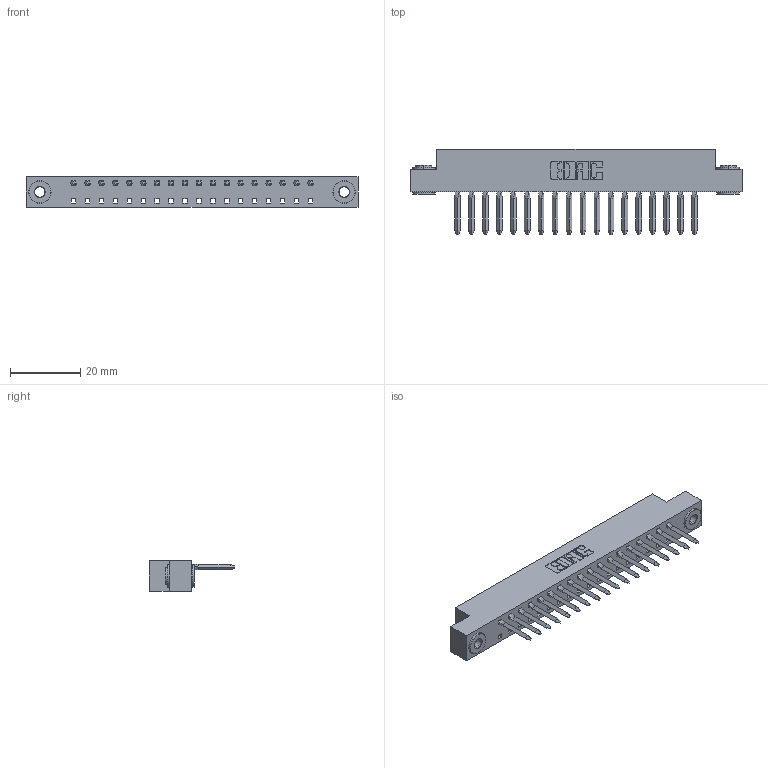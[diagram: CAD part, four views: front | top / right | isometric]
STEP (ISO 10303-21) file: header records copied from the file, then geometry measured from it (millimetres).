
FILE_DESCRIPTION (( 'STEP AP203' ), '1' );
FILE_NAME ('338-018-540-103.STEP', '2020-03-24T17:13:19', ( '' ), ( '' ), 'SwSTEP 2.0', 'SolidWorks 2016', '' );
FILE_SCHEMA (( 'CONFIG_CONTROL_DESIGN' ));
Length unit declared in the file: inch
Products named in the file (4): 338-290-001_540; 338-210-001_338-210-018-004; 345-250-002_345-250-002-102; 338-018-540-103
Assembly tree (21 placements, depth 2):
  338-018-540-103
    338-210-001_338-210-018-004
    338-290-001_540  x18
    345-250-002_345-250-002-102  x2
Bounding box: 94.34 x 24.21 x 8.71 mm (x, y, z)
Volume: 6439.2 mm3; surface area: 10164.1 mm2
Topology: 21 solids, 21 shells, 1820 faces, 4989 edges, 3190 vertices
Faces by surface type: plane 1244, cylinder 496, bspline 72, cone 8
Entity records: 38117 total; most frequent: CARTESIAN_POINT 7643, ORIENTED_EDGE 6400, DIRECTION 5989, EDGE_CURVE 3200, LINE 2357, VECTOR 2357, VERTEX_POINT 2078, AXIS2_PLACEMENT_3D 1816
